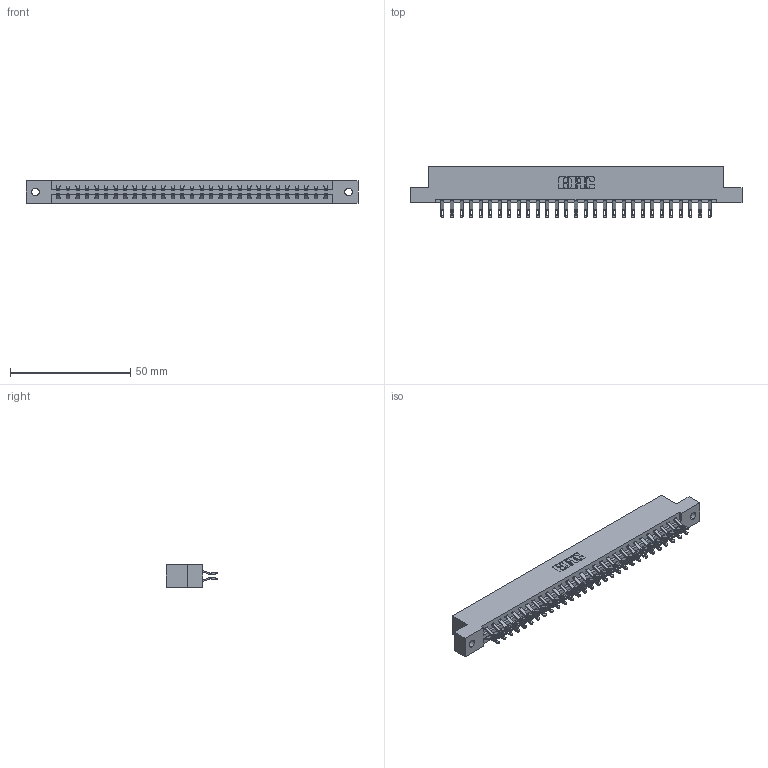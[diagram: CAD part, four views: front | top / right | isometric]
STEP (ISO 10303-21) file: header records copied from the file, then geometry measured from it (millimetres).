
FILE_DESCRIPTION (( 'STEP AP203' ), '1' );
FILE_NAME ('387-058-555-202.STEP', '2019-10-19T09:43:04', ( '' ), ( '' ), 'SwSTEP 2.0', 'SolidWorks 2016', '' );
FILE_SCHEMA (( 'CONFIG_CONTROL_DESIGN' ));
Length unit declared in the file: inch
Products named in the file (3): 337 Part_Flush Mounting Lugs - 0.128 Dia; 387-058-555-202; 345-292-001_555 Tail
Assembly tree (59 placements, depth 2):
  387-058-555-202
    337 Part_Flush Mounting Lugs - 0.128 Dia
    345-292-001_555 Tail  x58
Bounding box: 137.92 x 21.47 x 9.4 mm (x, y, z)
Volume: 14493.8 mm3; surface area: 16620.3 mm2
Topology: 59 solids, 59 shells, 3594 faces, 11273 edges, 7514 vertices
Faces by surface type: plane 2158, cylinder 1436
Entity records: 24495 total; most frequent: CARTESIAN_POINT 4172, ORIENTED_EDGE 4078, DIRECTION 3543, EDGE_CURVE 2039, VECTOR 1891, LINE 1891, VERTEX_POINT 1358, AXIS2_PLACEMENT_3D 826
